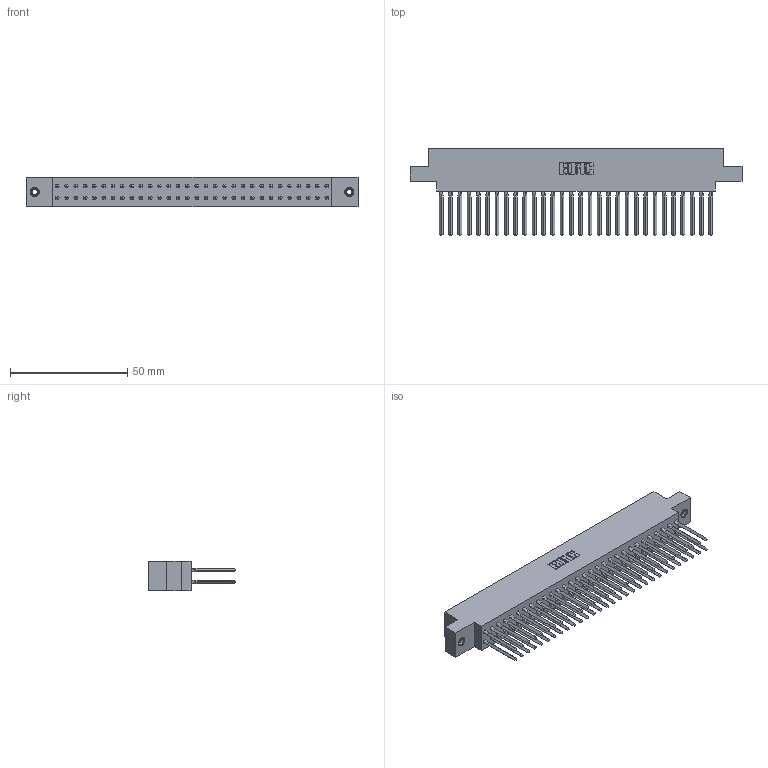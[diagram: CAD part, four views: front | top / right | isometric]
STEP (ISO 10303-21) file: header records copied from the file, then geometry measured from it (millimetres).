
FILE_DESCRIPTION (( 'STEP AP203' ), '1' );
FILE_NAME ('317-060-540-808.STEP', '2020-02-28T05:01:03', ( '' ), ( '' ), 'SwSTEP 2.0', 'SolidWorks 2016', '' );
FILE_SCHEMA (( 'CONFIG_CONTROL_DESIGN' ));
Length unit declared in the file: inch
Products named in the file (4): 317-290-001_540; 317 Part_.156 Dia - TI; 317-060-540-808; 345-250-001_345-250-003-102
Assembly tree (63 placements, depth 2):
  317-060-540-808
    317 Part_.156 Dia - TI
    317-290-001_540  x60
    345-250-001_345-250-003-102  x2
Bounding box: 141.58 x 37.34 x 12.7 mm (x, y, z)
Volume: 23349.2 mm3; surface area: 34380.6 mm2
Topology: 63 solids, 63 shells, 5502 faces, 15231 edges, 9806 vertices
Faces by surface type: plane 4470, cylinder 776, bspline 240, cone 12, torus 4
Entity records: 46225 total; most frequent: CARTESIAN_POINT 8450, ORIENTED_EDGE 7942, DIRECTION 6667, EDGE_CURVE 3971, VECTOR 3695, LINE 3695, VERTEX_POINT 2637, AXIS2_PLACEMENT_3D 1486
